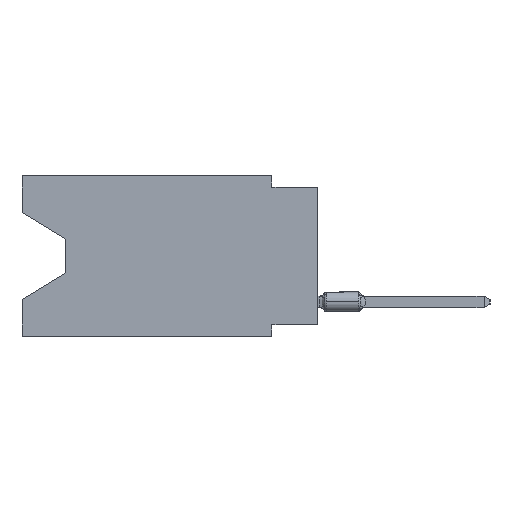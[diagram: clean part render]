
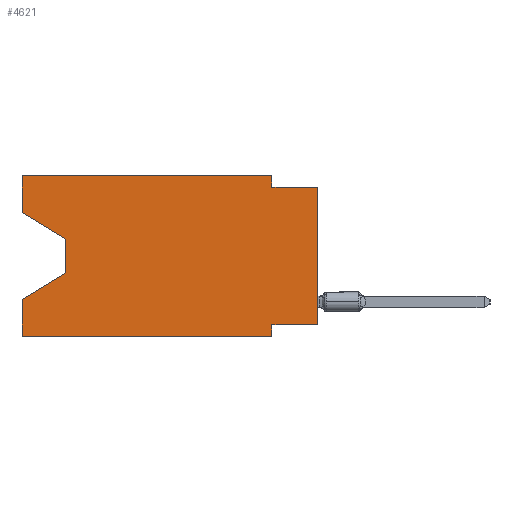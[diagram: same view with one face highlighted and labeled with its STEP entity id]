
A CAD part, left-side view. The second image highlights one B-rep face of the part: STEP entity #4621.
In plain terms, the highlighted planar face has unit normal (-1, 0, 0).
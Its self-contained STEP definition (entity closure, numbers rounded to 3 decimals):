
#757 = ORIENTED_EDGE ( 'NONE', *, *, #7671, .T. ) ;
#1008 = CARTESIAN_POINT ( 'NONE',  ( 0., 2.54, -8.89 ) ) ;
#1751 = CARTESIAN_POINT ( 'NONE',  ( 0., 16.383, -2.038 ) ) ;
#2513 = CARTESIAN_POINT ( 'NONE',  ( 0., 16.383, 0. ) ) ;
#3327 = ORIENTED_EDGE ( 'NONE', *, *, #10332, .T. ) ;
#4011 = VECTOR ( 'NONE', #28408, 1000. ) ;
#4256 = LINE ( 'NONE', #25859, #46333 ) ;
#4476 = CARTESIAN_POINT ( 'NONE',  ( 0., 16.383, 0. ) ) ;
#4621 = ADVANCED_FACE ( 'NONE', ( #20784 ), #13820, .F. ) ;
#5140 = LINE ( 'NONE', #35168, #4011 ) ;
#7387 = CARTESIAN_POINT ( 'NONE',  ( 0., 13.97, -5.385 ) ) ;
#7467 = DIRECTION ( 'NONE',  ( 0., 0., -1. ) ) ;
#7671 = EDGE_CURVE ( 'NONE', #41079, #7825, #12173, .T. ) ;
#7717 = ORIENTED_EDGE ( 'NONE', *, *, #8506, .F. ) ;
#7825 = VERTEX_POINT ( 'NONE', #38817 ) ;
#8506 = EDGE_CURVE ( 'NONE', #8545, #43839, #40506, .T. ) ;
#8545 = VERTEX_POINT ( 'NONE', #33783 ) ;
#9026 = CARTESIAN_POINT ( 'NONE',  ( 0., 16.383, 0. ) ) ;
#10059 = EDGE_CURVE ( 'NONE', #14086, #11355, #14058, .T. ) ;
#10073 = ORIENTED_EDGE ( 'NONE', *, *, #11022, .F. ) ;
#10208 = DIRECTION ( 'NONE',  ( 1., 0., 0. ) ) ;
#10332 = EDGE_CURVE ( 'NONE', #28153, #11355, #5140, .T. ) ;
#11022 = EDGE_CURVE ( 'NONE', #28153, #37206, #12278, .T. ) ;
#11355 = VERTEX_POINT ( 'NONE', #15571 ) ;
#11967 = EDGE_CURVE ( 'NONE', #32879, #41079, #25304, .T. ) ;
#11980 = VECTOR ( 'NONE', #7467, 1000. ) ;
#12173 = LINE ( 'NONE', #7387, #37543 ) ;
#12278 = LINE ( 'NONE', #34374, #28477 ) ;
#12288 = CARTESIAN_POINT ( 'NONE',  ( 0., 2.54, 0. ) ) ;
#12290 = VECTOR ( 'NONE', #43001, 1000. ) ;
#13401 = VECTOR ( 'NONE', #40562, 1000. ) ;
#13820 = PLANE ( 'NONE',  #31395 ) ;
#14055 = VECTOR ( 'NONE', #15781, 1000. ) ;
#14058 = LINE ( 'NONE', #14297, #30053 ) ;
#14086 = VERTEX_POINT ( 'NONE', #20486 ) ;
#14126 = DIRECTION ( 'NONE',  ( 0., -1., 0. ) ) ;
#14297 = CARTESIAN_POINT ( 'NONE',  ( 0., 0., -0.635 ) ) ;
#15225 = ORIENTED_EDGE ( 'NONE', *, *, #24897, .F. ) ;
#15452 = LINE ( 'NONE', #1008, #21209 ) ;
#15571 = CARTESIAN_POINT ( 'NONE',  ( 0., 0., -0.635 ) ) ;
#15781 = DIRECTION ( 'NONE',  ( 0., -1., 0. ) ) ;
#16744 = CARTESIAN_POINT ( 'NONE',  ( 0., 0., -8.255 ) ) ;
#16803 = CARTESIAN_POINT ( 'NONE',  ( 0., 13.97, -3.505 ) ) ;
#17762 = CARTESIAN_POINT ( 'NONE',  ( 0., 2.54, -8.89 ) ) ;
#18063 = CARTESIAN_POINT ( 'NONE',  ( 0., 2.54, -8.255 ) ) ;
#18859 = ORIENTED_EDGE ( 'NONE', *, *, #27411, .T. ) ;
#19091 = ORIENTED_EDGE ( 'NONE', *, *, #21744, .F. ) ;
#19772 = ORIENTED_EDGE ( 'NONE', *, *, #33086, .T. ) ;
#20349 = VERTEX_POINT ( 'NONE', #27953 ) ;
#20486 = CARTESIAN_POINT ( 'NONE',  ( 0., 2.54, -0.635 ) ) ;
#20784 = FACE_OUTER_BOUND ( 'NONE', #21232, .T. ) ;
#21209 = VECTOR ( 'NONE', #37551, 1000. ) ;
#21232 = EDGE_LOOP ( 'NONE', ( #18859, #23650, #757, #38797, #19772, #15225, #10073, #3327, #24649, #44415, #19091, #7717 ) ) ;
#21744 = EDGE_CURVE ( 'NONE', #43839, #26057, #27777, .T. ) ;
#23055 = DIRECTION ( 'NONE',  ( 0., 1., 0. ) ) ;
#23650 = ORIENTED_EDGE ( 'NONE', *, *, #11967, .T. ) ;
#24649 = ORIENTED_EDGE ( 'NONE', *, *, #10059, .F. ) ;
#24831 = DIRECTION ( 'NONE',  ( 0., 0., -1. ) ) ;
#24897 = EDGE_CURVE ( 'NONE', #37206, #33699, #15452, .T. ) ;
#25304 = LINE ( 'NONE', #33021, #29304 ) ;
#25859 = CARTESIAN_POINT ( 'NONE',  ( 0., 16.383, -8.89 ) ) ;
#26057 = VERTEX_POINT ( 'NONE', #12288 ) ;
#27057 = CARTESIAN_POINT ( 'NONE',  ( 0., 16.383, 0. ) ) ;
#27411 = EDGE_CURVE ( 'NONE', #8545, #32879, #28345, .T. ) ;
#27777 = LINE ( 'NONE', #27057, #14055 ) ;
#27953 = CARTESIAN_POINT ( 'NONE',  ( 0., 16.383, -8.89 ) ) ;
#28153 = VERTEX_POINT ( 'NONE', #16744 ) ;
#28345 = LINE ( 'NONE', #1751, #12290 ) ;
#28408 = DIRECTION ( 'NONE',  ( 0., 0., 1. ) ) ;
#28477 = VECTOR ( 'NONE', #23055, 1000. ) ;
#29304 = VECTOR ( 'NONE', #39983, 1000. ) ;
#29548 = CARTESIAN_POINT ( 'NONE',  ( 0., 2.54, 0. ) ) ;
#30053 = VECTOR ( 'NONE', #46719, 1000. ) ;
#31395 = AXIS2_PLACEMENT_3D ( 'NONE', #2513, #10208, #24831 ) ;
#32879 = VERTEX_POINT ( 'NONE', #16803 ) ;
#33021 = CARTESIAN_POINT ( 'NONE',  ( 0., 13.97, -3.505 ) ) ;
#33086 = EDGE_CURVE ( 'NONE', #20349, #33699, #4256, .T. ) ;
#33699 = VERTEX_POINT ( 'NONE', #17762 ) ;
#33783 = CARTESIAN_POINT ( 'NONE',  ( 0., 16.383, -2.038 ) ) ;
#34374 = CARTESIAN_POINT ( 'NONE',  ( 0., 0., -8.255 ) ) ;
#35168 = CARTESIAN_POINT ( 'NONE',  ( 0., 0., 0. ) ) ;
#36690 = DIRECTION ( 'NONE',  ( 0., 0.855, -0.519 ) ) ;
#36866 = VECTOR ( 'NONE', #44804, 1000. ) ;
#36960 = CARTESIAN_POINT ( 'NONE',  ( 0., 16.383, 0. ) ) ;
#37206 = VERTEX_POINT ( 'NONE', #18063 ) ;
#37543 = VECTOR ( 'NONE', #36690, 1000. ) ;
#37551 = DIRECTION ( 'NONE',  ( 0., 0., -1. ) ) ;
#37568 = EDGE_CURVE ( 'NONE', #20349, #7825, #47541, .T. ) ;
#38797 = ORIENTED_EDGE ( 'NONE', *, *, #37568, .F. ) ;
#38817 = CARTESIAN_POINT ( 'NONE',  ( 0., 16.383, -6.852 ) ) ;
#39922 = CARTESIAN_POINT ( 'NONE',  ( 0., 13.97, -5.385 ) ) ;
#39983 = DIRECTION ( 'NONE',  ( 0., 0., -1. ) ) ;
#40506 = LINE ( 'NONE', #4476, #36866 ) ;
#40562 = DIRECTION ( 'NONE',  ( 0., 0., 1. ) ) ;
#41079 = VERTEX_POINT ( 'NONE', #39922 ) ;
#41410 = EDGE_CURVE ( 'NONE', #26057, #14086, #43950, .T. ) ;
#43001 = DIRECTION ( 'NONE',  ( 0., -0.855, -0.519 ) ) ;
#43839 = VERTEX_POINT ( 'NONE', #9026 ) ;
#43950 = LINE ( 'NONE', #29548, #11980 ) ;
#44415 = ORIENTED_EDGE ( 'NONE', *, *, #41410, .F. ) ;
#44804 = DIRECTION ( 'NONE',  ( 0., 0., 1. ) ) ;
#46333 = VECTOR ( 'NONE', #14126, 1000. ) ;
#46719 = DIRECTION ( 'NONE',  ( 0., -1., 0. ) ) ;
#47541 = LINE ( 'NONE', #36960, #13401 ) ;
